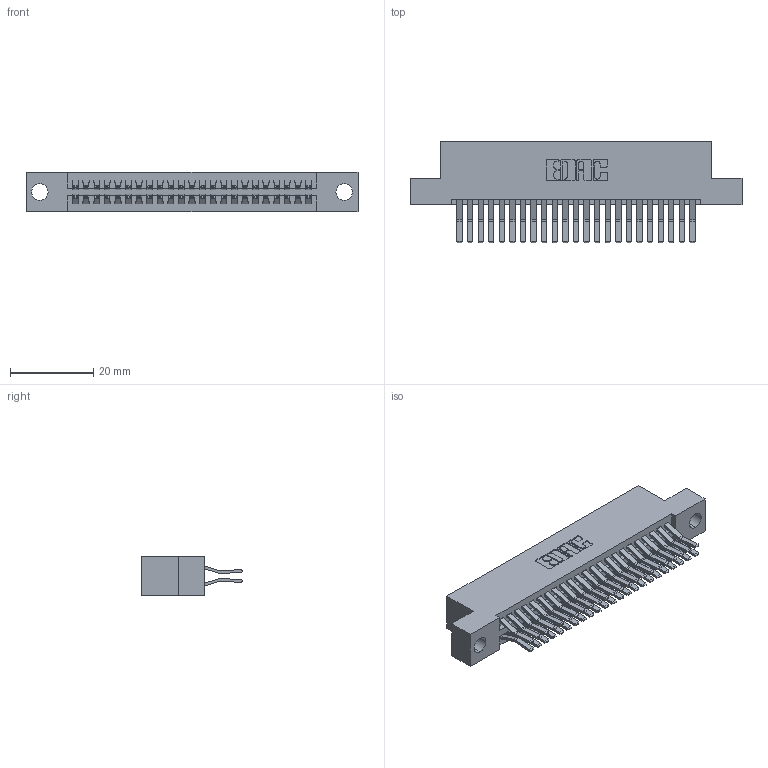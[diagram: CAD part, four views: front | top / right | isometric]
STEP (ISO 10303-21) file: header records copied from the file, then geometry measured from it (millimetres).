
FILE_DESCRIPTION (( 'STEP AP203' ), '1' );
FILE_NAME ('345-046-560-204.STEP', '2021-05-20T02:35:22', ( '' ), ( '' ), 'SwSTEP 2.0', 'SolidWorks 2020', '' );
FILE_SCHEMA (( 'CONFIG_CONTROL_DESIGN' ));
Length unit declared in the file: inch
Products named in the file (3): 345-046-560-204; 345-292-001_560 Tail; 345 Part_Flush Mounting Lugs - 0.156 Dia-TI
Assembly tree (47 placements, depth 2):
  345-046-560-204
    345 Part_Flush Mounting Lugs - 0.156 Dia-TI
    345-292-001_560 Tail  x46
Bounding box: 79.63 x 24.45 x 9.4 mm (x, y, z)
Volume: 7754.4 mm3; surface area: 11721.4 mm2
Topology: 47 solids, 47 shells, 2532 faces, 7507 edges, 4942 vertices
Faces by surface type: plane 1612, cylinder 920
Entity records: 21111 total; most frequent: CARTESIAN_POINT 3562, ORIENTED_EDGE 3494, DIRECTION 3167, EDGE_CURVE 1747, VECTOR 1519, LINE 1519, VERTEX_POINT 1162, AXIS2_PLACEMENT_3D 824
